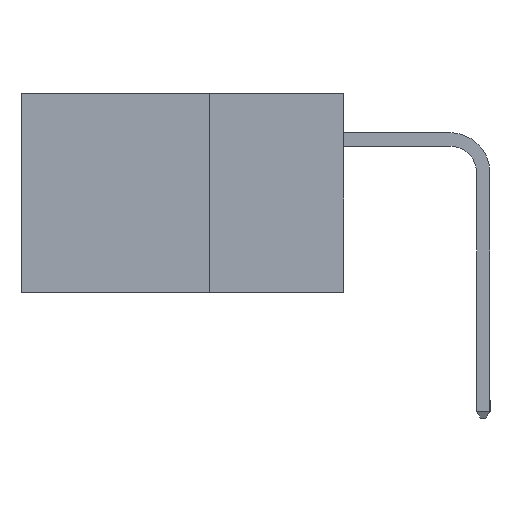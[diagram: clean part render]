
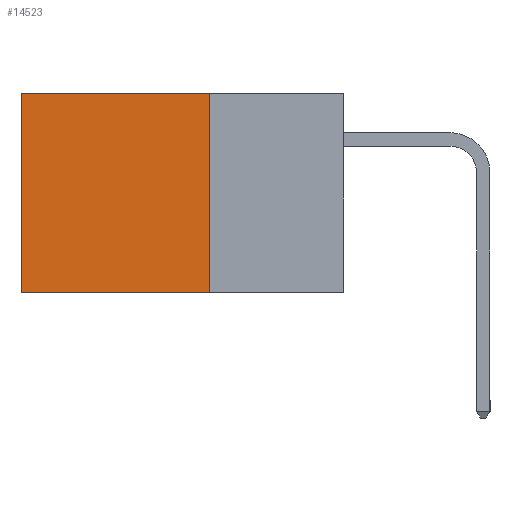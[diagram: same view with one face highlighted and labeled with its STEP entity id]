
A CAD part, left-side view. The second image highlights one B-rep face of the part: STEP entity #14523.
In plain terms, the highlighted planar face has unit normal (-1, 0, 0).
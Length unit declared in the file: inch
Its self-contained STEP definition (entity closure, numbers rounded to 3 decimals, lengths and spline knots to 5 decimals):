
#189 = DIRECTION ( 'NONE',  ( 1., 0., 0. ) ) ;
#487 = CARTESIAN_POINT ( 'NONE',  ( 0.2615, 0.25, 0. ) ) ;
#680 = LINE ( 'NONE', #2970, #11594 ) ;
#747 = VECTOR ( 'NONE', #3059, 39.37008 ) ;
#1492 = ORIENTED_EDGE ( 'NONE', *, *, #1797, .T. ) ;
#1672 = DIRECTION ( 'NONE',  ( 0., 1., 0. ) ) ;
#1753 = EDGE_CURVE ( 'NONE', #3115, #4032, #4607, .T. ) ;
#1797 = EDGE_CURVE ( 'NONE', #5971, #5316, #7966, .T. ) ;
#2970 = CARTESIAN_POINT ( 'NONE',  ( 0.2615, 0.25, -0.37 ) ) ;
#3059 = DIRECTION ( 'NONE',  ( 0., 1., 0. ) ) ;
#3115 = VERTEX_POINT ( 'NONE', #7804 ) ;
#3961 = ORIENTED_EDGE ( 'NONE', *, *, #1753, .F. ) ;
#4032 = VERTEX_POINT ( 'NONE', #11011 ) ;
#4248 = EDGE_CURVE ( 'NONE', #5971, #3115, #680, .T. ) ;
#4438 = DIRECTION ( 'NONE',  ( 0., 0., -1. ) ) ;
#4602 = FACE_OUTER_BOUND ( 'NONE', #17653, .T. ) ;
#4607 = LINE ( 'NONE', #7346, #747 ) ;
#5316 = VERTEX_POINT ( 'NONE', #15762 ) ;
#5971 = VERTEX_POINT ( 'NONE', #487 ) ;
#7346 = CARTESIAN_POINT ( 'NONE',  ( 0.2615, 0.25, -0.37 ) ) ;
#7522 = VECTOR ( 'NONE', #1672, 39.37008 ) ;
#7804 = CARTESIAN_POINT ( 'NONE',  ( 0.2615, 0.25, -0.37 ) ) ;
#7966 = LINE ( 'NONE', #10263, #7522 ) ;
#8814 = CARTESIAN_POINT ( 'NONE',  ( 0.2615, 0.25, -0.37 ) ) ;
#10199 = DIRECTION ( 'NONE',  ( 0., 0., -1. ) ) ;
#10263 = CARTESIAN_POINT ( 'NONE',  ( 0.2615, 0.25, 0. ) ) ;
#11011 = CARTESIAN_POINT ( 'NONE',  ( 0.2615, 0.6, -0.37 ) ) ;
#11594 = VECTOR ( 'NONE', #4438, 39.37008 ) ;
#13130 = LINE ( 'NONE', #16357, #15948 ) ;
#13637 = DIRECTION ( 'NONE',  ( 0., 0., -1. ) ) ;
#14523 = ADVANCED_FACE ( 'NONE', ( #4602 ), #17119, .F. ) ;
#14798 = AXIS2_PLACEMENT_3D ( 'NONE', #8814, #189, #10199 ) ;
#15065 = ORIENTED_EDGE ( 'NONE', *, *, #15486, .T. ) ;
#15141 = ORIENTED_EDGE ( 'NONE', *, *, #4248, .F. ) ;
#15486 = EDGE_CURVE ( 'NONE', #5316, #4032, #13130, .T. ) ;
#15762 = CARTESIAN_POINT ( 'NONE',  ( 0.2615, 0.6, 0. ) ) ;
#15948 = VECTOR ( 'NONE', #13637, 39.37008 ) ;
#16357 = CARTESIAN_POINT ( 'NONE',  ( 0.2615, 0.6, -0.37 ) ) ;
#17119 = PLANE ( 'NONE',  #14798 ) ;
#17653 = EDGE_LOOP ( 'NONE', ( #15065, #3961, #15141, #1492 ) ) ;
